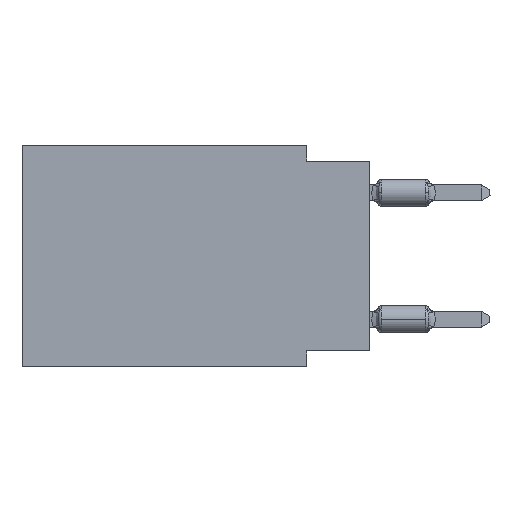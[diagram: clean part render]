
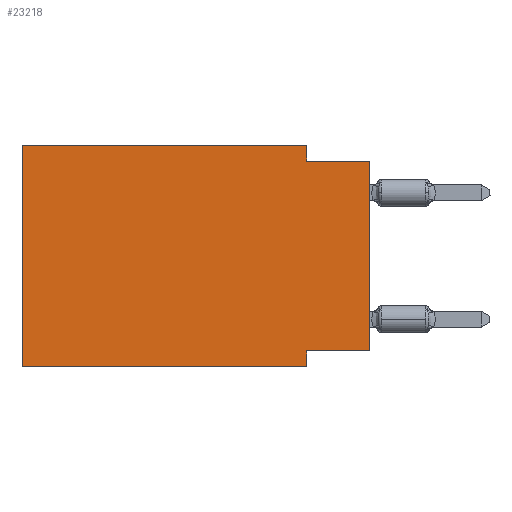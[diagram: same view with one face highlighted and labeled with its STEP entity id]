
A CAD part, left-side view. The second image highlights one B-rep face of the part: STEP entity #23218.
In plain terms, the highlighted planar face has unit normal (-1, 0, 0).
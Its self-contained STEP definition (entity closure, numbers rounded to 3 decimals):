
#455 = DIRECTION ( 'NONE',  ( 0., -1., 0. ) ) ;
#2083 = PLANE ( 'NONE',  #16100 ) ;
#2437 = EDGE_CURVE ( 'NONE', #5499, #29330, #33735, .T. ) ;
#2602 = DIRECTION ( 'NONE',  ( 0., 0., 1. ) ) ;
#2775 = CARTESIAN_POINT ( 'NONE',  ( 0., 2.54, -0.635 ) ) ;
#5230 = DIRECTION ( 'NONE',  ( 1., 0., 0. ) ) ;
#5499 = VERTEX_POINT ( 'NONE', #2775 ) ;
#6127 = ORIENTED_EDGE ( 'NONE', *, *, #14514, .T. ) ;
#6721 = CARTESIAN_POINT ( 'NONE',  ( 0., 13.97, -8.89 ) ) ;
#6838 = VECTOR ( 'NONE', #2602, 1000. ) ;
#7346 = CARTESIAN_POINT ( 'NONE',  ( 0., 13.97, -8.89 ) ) ;
#7468 = CARTESIAN_POINT ( 'NONE',  ( 0., 0., -8.255 ) ) ;
#7857 = EDGE_CURVE ( 'NONE', #25881, #28901, #10770, .T. ) ;
#9169 = EDGE_CURVE ( 'NONE', #15152, #5499, #40048, .T. ) ;
#10231 = VERTEX_POINT ( 'NONE', #7468 ) ;
#10712 = CARTESIAN_POINT ( 'NONE',  ( 0., 13.97, 0. ) ) ;
#10770 = LINE ( 'NONE', #24352, #31319 ) ;
#11683 = CARTESIAN_POINT ( 'NONE',  ( 0., 13.97, 0. ) ) ;
#12684 = EDGE_CURVE ( 'NONE', #10231, #29330, #34780, .T. ) ;
#13077 = EDGE_LOOP ( 'NONE', ( #25851, #15278, #27291, #20288, #37990, #6127, #19288, #15631 ) ) ;
#14112 = DIRECTION ( 'NONE',  ( 0., 0., -1. ) ) ;
#14407 = VERTEX_POINT ( 'NONE', #6721 ) ;
#14514 = EDGE_CURVE ( 'NONE', #14407, #28901, #29108, .T. ) ;
#14598 = DIRECTION ( 'NONE',  ( 0., 0., -1. ) ) ;
#14599 = LINE ( 'NONE', #27359, #27984 ) ;
#15092 = VECTOR ( 'NONE', #34546, 1000. ) ;
#15152 = VERTEX_POINT ( 'NONE', #17565 ) ;
#15278 = ORIENTED_EDGE ( 'NONE', *, *, #2437, .F. ) ;
#15631 = ORIENTED_EDGE ( 'NONE', *, *, #30639, .F. ) ;
#16100 = AXIS2_PLACEMENT_3D ( 'NONE', #18826, #5230, #33863 ) ;
#17565 = CARTESIAN_POINT ( 'NONE',  ( 0., 2.54, 0. ) ) ;
#18826 = CARTESIAN_POINT ( 'NONE',  ( 0., 13.97, 0. ) ) ;
#19288 = ORIENTED_EDGE ( 'NONE', *, *, #7857, .F. ) ;
#20269 = CARTESIAN_POINT ( 'NONE',  ( 0., 2.54, -8.255 ) ) ;
#20288 = ORIENTED_EDGE ( 'NONE', *, *, #22133, .F. ) ;
#20372 = CARTESIAN_POINT ( 'NONE',  ( 0., 13.97, 0. ) ) ;
#22133 = EDGE_CURVE ( 'NONE', #27748, #15152, #36594, .T. ) ;
#23218 = ADVANCED_FACE ( 'NONE', ( #27823 ), #2083, .F. ) ;
#23775 = VECTOR ( 'NONE', #35444, 1000. ) ;
#23886 = DIRECTION ( 'NONE',  ( 0., -1., 0. ) ) ;
#24352 = CARTESIAN_POINT ( 'NONE',  ( 0., 2.54, -8.89 ) ) ;
#25851 = ORIENTED_EDGE ( 'NONE', *, *, #12684, .T. ) ;
#25881 = VERTEX_POINT ( 'NONE', #20269 ) ;
#27291 = ORIENTED_EDGE ( 'NONE', *, *, #9169, .F. ) ;
#27292 = CARTESIAN_POINT ( 'NONE',  ( 0., 0., -0.635 ) ) ;
#27359 = CARTESIAN_POINT ( 'NONE',  ( 0., 0., -8.255 ) ) ;
#27748 = VERTEX_POINT ( 'NONE', #11683 ) ;
#27823 = FACE_OUTER_BOUND ( 'NONE', #13077, .T. ) ;
#27905 = EDGE_CURVE ( 'NONE', #14407, #27748, #29991, .T. ) ;
#27934 = CARTESIAN_POINT ( 'NONE',  ( 0., 0., 0. ) ) ;
#27984 = VECTOR ( 'NONE', #36914, 1000. ) ;
#28901 = VERTEX_POINT ( 'NONE', #29887 ) ;
#29108 = LINE ( 'NONE', #7346, #30352 ) ;
#29330 = VERTEX_POINT ( 'NONE', #33371 ) ;
#29887 = CARTESIAN_POINT ( 'NONE',  ( 0., 2.54, -8.89 ) ) ;
#29991 = LINE ( 'NONE', #20372, #23775 ) ;
#30352 = VECTOR ( 'NONE', #455, 1000. ) ;
#30476 = CARTESIAN_POINT ( 'NONE',  ( 0., 2.54, 0. ) ) ;
#30639 = EDGE_CURVE ( 'NONE', #10231, #25881, #14599, .T. ) ;
#31319 = VECTOR ( 'NONE', #14112, 1000. ) ;
#31385 = VECTOR ( 'NONE', #23886, 1000. ) ;
#33371 = CARTESIAN_POINT ( 'NONE',  ( 0., 0., -0.635 ) ) ;
#33735 = LINE ( 'NONE', #27292, #15092 ) ;
#33863 = DIRECTION ( 'NONE',  ( 0., 0., -1. ) ) ;
#34079 = VECTOR ( 'NONE', #14598, 1000. ) ;
#34546 = DIRECTION ( 'NONE',  ( 0., -1., 0. ) ) ;
#34780 = LINE ( 'NONE', #27934, #6838 ) ;
#35444 = DIRECTION ( 'NONE',  ( 0., 0., 1. ) ) ;
#36594 = LINE ( 'NONE', #10712, #31385 ) ;
#36914 = DIRECTION ( 'NONE',  ( 0., 1., 0. ) ) ;
#37990 = ORIENTED_EDGE ( 'NONE', *, *, #27905, .F. ) ;
#40048 = LINE ( 'NONE', #30476, #34079 ) ;
